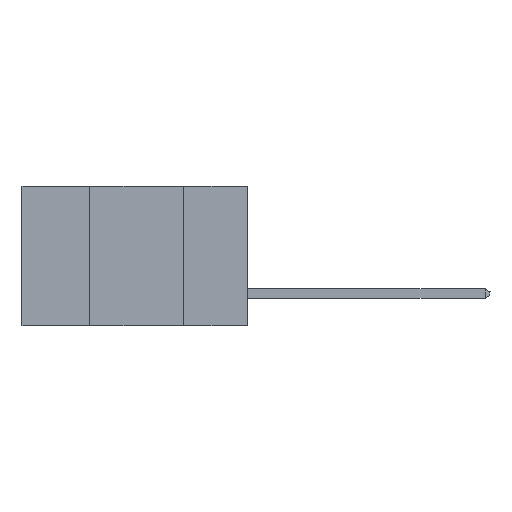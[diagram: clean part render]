
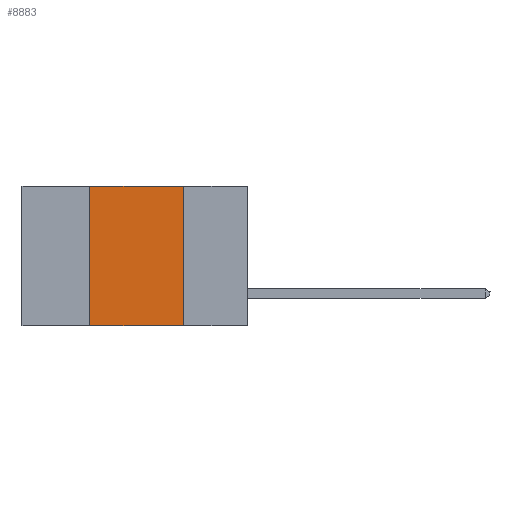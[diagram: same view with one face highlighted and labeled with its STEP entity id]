
A CAD part, left-side view. The second image highlights one B-rep face of the part: STEP entity #8883.
In plain terms, the highlighted planar face has unit normal (-1, 0, 0).
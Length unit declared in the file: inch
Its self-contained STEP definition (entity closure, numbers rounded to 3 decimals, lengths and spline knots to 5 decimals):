
#449 = VERTEX_POINT ( 'NONE', #11382 ) ;
#653 = EDGE_LOOP ( 'NONE', ( #3589, #8227, #3952, #6728 ) ) ;
#726 = PLANE ( 'NONE',  #768 ) ;
#768 = AXIS2_PLACEMENT_3D ( 'NONE', #7230, #11034, #7290 ) ;
#1020 = CARTESIAN_POINT ( 'NONE',  ( 0., 0.6, 0. ) ) ;
#1253 = CARTESIAN_POINT ( 'NONE',  ( 0., 0.17, 0. ) ) ;
#1380 = LINE ( 'NONE', #11811, #11568 ) ;
#1693 = CARTESIAN_POINT ( 'NONE',  ( 0., 0.42, -0.37 ) ) ;
#2143 = VECTOR ( 'NONE', #2843, 39.37008 ) ;
#2679 = EDGE_CURVE ( 'NONE', #6807, #449, #11157, .T. ) ;
#2843 = DIRECTION ( 'NONE',  ( 0., -1., 0. ) ) ;
#3589 = ORIENTED_EDGE ( 'NONE', *, *, #4445, .F. ) ;
#3952 = ORIENTED_EDGE ( 'NONE', *, *, #2679, .F. ) ;
#4155 = EDGE_CURVE ( 'NONE', #449, #5408, #9587, .T. ) ;
#4421 = VECTOR ( 'NONE', #8128, 39.37008 ) ;
#4445 = EDGE_CURVE ( 'NONE', #5408, #11823, #7251, .T. ) ;
#5408 = VERTEX_POINT ( 'NONE', #1253 ) ;
#6377 = CARTESIAN_POINT ( 'NONE',  ( 0., 0.17, -0.37 ) ) ;
#6636 = VECTOR ( 'NONE', #9292, 39.37008 ) ;
#6728 = ORIENTED_EDGE ( 'NONE', *, *, #10189, .T. ) ;
#6807 = VERTEX_POINT ( 'NONE', #1693 ) ;
#7230 = CARTESIAN_POINT ( 'NONE',  ( 0., 0.6, 0. ) ) ;
#7251 = LINE ( 'NONE', #6377, #4421 ) ;
#7290 = DIRECTION ( 'NONE',  ( 0., 0., -1. ) ) ;
#7945 = DIRECTION ( 'NONE',  ( 0., -1., 0. ) ) ;
#8128 = DIRECTION ( 'NONE',  ( 0., 0., -1. ) ) ;
#8227 = ORIENTED_EDGE ( 'NONE', *, *, #4155, .F. ) ;
#8409 = CARTESIAN_POINT ( 'NONE',  ( 0., 0.42, -0.37 ) ) ;
#8883 = ADVANCED_FACE ( 'NONE', ( #10231 ), #726, .F. ) ;
#9292 = DIRECTION ( 'NONE',  ( 0., 0., 1. ) ) ;
#9587 = LINE ( 'NONE', #1020, #2143 ) ;
#10189 = EDGE_CURVE ( 'NONE', #6807, #11823, #1380, .T. ) ;
#10231 = FACE_OUTER_BOUND ( 'NONE', #653, .T. ) ;
#11034 = DIRECTION ( 'NONE',  ( 1., 0., 0. ) ) ;
#11157 = LINE ( 'NONE', #8409, #6636 ) ;
#11382 = CARTESIAN_POINT ( 'NONE',  ( 0., 0.42, 0. ) ) ;
#11512 = CARTESIAN_POINT ( 'NONE',  ( 0., 0.17, -0.37 ) ) ;
#11568 = VECTOR ( 'NONE', #7945, 39.37008 ) ;
#11811 = CARTESIAN_POINT ( 'NONE',  ( 0., 0.6, -0.37 ) ) ;
#11823 = VERTEX_POINT ( 'NONE', #11512 ) ;
